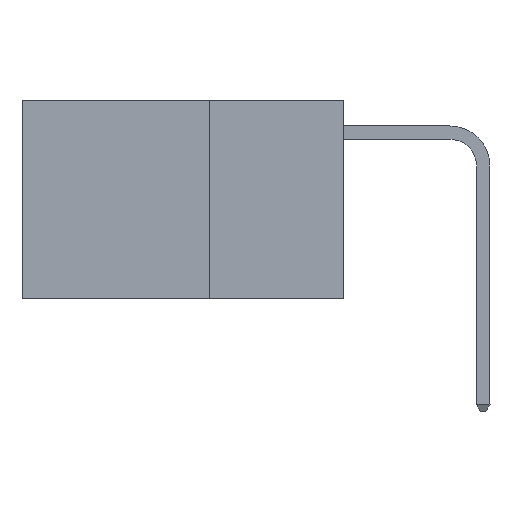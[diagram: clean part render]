
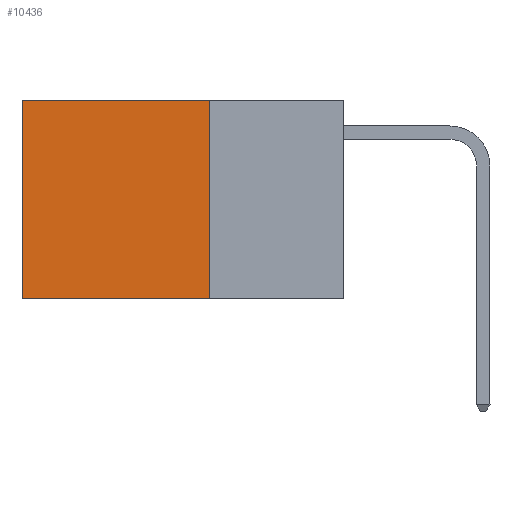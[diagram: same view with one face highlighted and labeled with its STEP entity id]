
A CAD part, left-side view. The second image highlights one B-rep face of the part: STEP entity #10436.
In plain terms, the highlighted planar face has unit normal (-1, 0, 0).
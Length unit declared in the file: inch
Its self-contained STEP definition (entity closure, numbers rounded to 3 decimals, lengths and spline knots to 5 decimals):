
#178 = LINE ( 'NONE', #7272, #9325 ) ;
#223 = VERTEX_POINT ( 'NONE', #4884 ) ;
#1199 = VERTEX_POINT ( 'NONE', #21420 ) ;
#1415 = EDGE_CURVE ( 'NONE', #20959, #223, #17585, .T. ) ;
#4884 = CARTESIAN_POINT ( 'NONE',  ( 0.2625, 0.6, -0.37 ) ) ;
#5125 = VECTOR ( 'NONE', #7572, 39.37008 ) ;
#5346 = LINE ( 'NONE', #14656, #11616 ) ;
#6191 = FACE_OUTER_BOUND ( 'NONE', #13413, .T. ) ;
#7272 = CARTESIAN_POINT ( 'NONE',  ( 0.2625, 0.25, 0. ) ) ;
#7497 = ORIENTED_EDGE ( 'NONE', *, *, #8149, .F. ) ;
#7572 = DIRECTION ( 'NONE',  ( 0., 1., 0. ) ) ;
#7930 = CARTESIAN_POINT ( 'NONE',  ( 0.2625, 0.25, 0. ) ) ;
#8149 = EDGE_CURVE ( 'NONE', #1199, #9626, #178, .T. ) ;
#9320 = EDGE_CURVE ( 'NONE', #1199, #20959, #5346, .T. ) ;
#9325 = VECTOR ( 'NONE', #14394, 39.37008 ) ;
#9626 = VERTEX_POINT ( 'NONE', #9960 ) ;
#9960 = CARTESIAN_POINT ( 'NONE',  ( 0.2625, 0.25, -0.37 ) ) ;
#10270 = CARTESIAN_POINT ( 'NONE',  ( 0.2625, 0.6, 0. ) ) ;
#10436 = ADVANCED_FACE ( 'NONE', ( #6191 ), #22121, .F. ) ;
#11082 = CARTESIAN_POINT ( 'NONE',  ( 0.2625, 0.6, 0. ) ) ;
#11616 = VECTOR ( 'NONE', #12444, 39.37008 ) ;
#12025 = DIRECTION ( 'NONE',  ( 0., 0., -1. ) ) ;
#12444 = DIRECTION ( 'NONE',  ( 0., 1., 0. ) ) ;
#13185 = DIRECTION ( 'NONE',  ( 1., 0., 0. ) ) ;
#13301 = DIRECTION ( 'NONE',  ( 0., 0., -1. ) ) ;
#13413 = EDGE_LOOP ( 'NONE', ( #19457, #16083, #7497, #13832 ) ) ;
#13832 = ORIENTED_EDGE ( 'NONE', *, *, #9320, .T. ) ;
#14394 = DIRECTION ( 'NONE',  ( 0., 0., -1. ) ) ;
#14656 = CARTESIAN_POINT ( 'NONE',  ( 0.2625, 0.25, 0. ) ) ;
#16083 = ORIENTED_EDGE ( 'NONE', *, *, #19804, .F. ) ;
#16644 = CARTESIAN_POINT ( 'NONE',  ( 0.2625, 0.25, -0.37 ) ) ;
#17585 = LINE ( 'NONE', #10270, #22214 ) ;
#18251 = AXIS2_PLACEMENT_3D ( 'NONE', #7930, #13185, #13301 ) ;
#19457 = ORIENTED_EDGE ( 'NONE', *, *, #1415, .T. ) ;
#19804 = EDGE_CURVE ( 'NONE', #9626, #223, #22307, .T. ) ;
#20959 = VERTEX_POINT ( 'NONE', #11082 ) ;
#21420 = CARTESIAN_POINT ( 'NONE',  ( 0.2625, 0.25, 0. ) ) ;
#22121 = PLANE ( 'NONE',  #18251 ) ;
#22214 = VECTOR ( 'NONE', #12025, 39.37008 ) ;
#22307 = LINE ( 'NONE', #16644, #5125 ) ;
